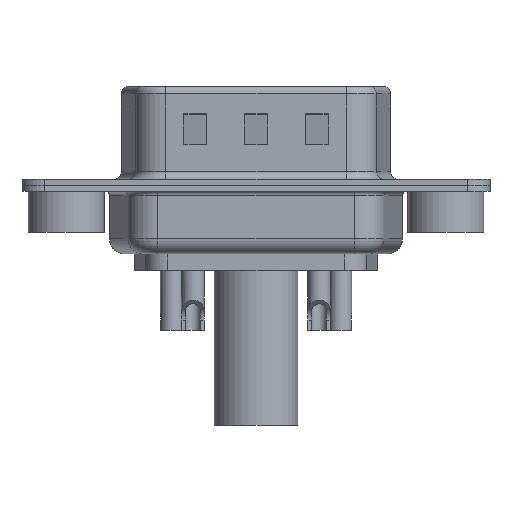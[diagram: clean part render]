
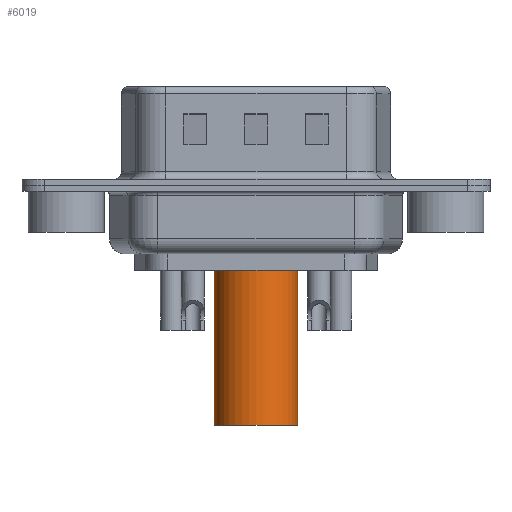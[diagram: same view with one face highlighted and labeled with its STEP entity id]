
A CAD part, front view. The second image highlights one B-rep face of the part: STEP entity #6019.
In plain terms, the highlighted cylindrical face has radius 2.75 mm (diameter 5.5 mm), a partial arc.
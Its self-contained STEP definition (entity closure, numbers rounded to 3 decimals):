
#154 = LINE ( 'NONE', #9573, #10077 ) ;
#379 = LINE ( 'NONE', #12700, #9889 ) ;
#721 = LINE ( 'NONE', #5029, #2576 ) ;
#1055 = CARTESIAN_POINT ( 'NONE',  ( 2.75, 0., -7.764 ) ) ;
#1066 = CARTESIAN_POINT ( 'NONE',  ( -2.75, 0., 1.5 ) ) ;
#1261 = VERTEX_POINT ( 'NONE', #1055 ) ;
#1787 = CYLINDRICAL_SURFACE ( 'NONE', #6380, 2.75 ) ;
#2061 = VERTEX_POINT ( 'NONE', #14835 ) ;
#2210 = DIRECTION ( 'NONE',  ( 1., 0., 0. ) ) ;
#2412 = VERTEX_POINT ( 'NONE', #3346 ) ;
#2435 = CARTESIAN_POINT ( 'NONE',  ( 0., 0., -8.7 ) ) ;
#2576 = VECTOR ( 'NONE', #14146, 1000. ) ;
#3346 = CARTESIAN_POINT ( 'NONE',  ( -2.75, 0., -7.764 ) ) ;
#3786 = CIRCLE ( 'NONE', #8337, 2.75 ) ;
#3791 = EDGE_CURVE ( 'NONE', #16579, #5732, #16949, .T. ) ;
#4065 = EDGE_CURVE ( 'NONE', #2412, #14189, #379, .T. ) ;
#4351 = EDGE_CURVE ( 'NONE', #1261, #5732, #154, .T. ) ;
#4930 = EDGE_CURVE ( 'NONE', #2412, #16579, #7479, .T. ) ;
#5029 = CARTESIAN_POINT ( 'NONE',  ( 2.75, 0., 4.234 ) ) ;
#5094 = CARTESIAN_POINT ( 'NONE',  ( 0., 0., 1.5 ) ) ;
#5098 = EDGE_LOOP ( 'NONE', ( #8766, #8073, #16456, #15986, #11383, #16383 ) ) ;
#5732 = VERTEX_POINT ( 'NONE', #8247 ) ;
#6019 = ADVANCED_FACE ( 'NONE', ( #16147 ), #1787, .T. ) ;
#6376 = DIRECTION ( 'NONE',  ( 1., 0., 0. ) ) ;
#6380 = AXIS2_PLACEMENT_3D ( 'NONE', #8889, #12108, #7188 ) ;
#6591 = EDGE_CURVE ( 'NONE', #14189, #2061, #3786, .T. ) ;
#7188 = DIRECTION ( 'NONE',  ( 1., 0., 0. ) ) ;
#7245 = CARTESIAN_POINT ( 'NONE',  ( -2.75, 0., -8.7 ) ) ;
#7479 = LINE ( 'NONE', #9342, #14003 ) ;
#7665 = AXIS2_PLACEMENT_3D ( 'NONE', #2435, #12833, #2210 ) ;
#8073 = ORIENTED_EDGE ( 'NONE', *, *, #4930, .T. ) ;
#8247 = CARTESIAN_POINT ( 'NONE',  ( 2.75, 0., -8.7 ) ) ;
#8337 = AXIS2_PLACEMENT_3D ( 'NONE', #5094, #14232, #6376 ) ;
#8502 = DIRECTION ( 'NONE',  ( 0., 0., -1. ) ) ;
#8766 = ORIENTED_EDGE ( 'NONE', *, *, #4065, .F. ) ;
#8889 = CARTESIAN_POINT ( 'NONE',  ( 0., 0., 4.234 ) ) ;
#9342 = CARTESIAN_POINT ( 'NONE',  ( -2.75, 0., -8.7 ) ) ;
#9573 = CARTESIAN_POINT ( 'NONE',  ( 2.75, 0., -8.7 ) ) ;
#9889 = VECTOR ( 'NONE', #11554, 1000. ) ;
#10077 = VECTOR ( 'NONE', #8502, 1000. ) ;
#11383 = ORIENTED_EDGE ( 'NONE', *, *, #14953, .T. ) ;
#11554 = DIRECTION ( 'NONE',  ( 0., 0., 1. ) ) ;
#12108 = DIRECTION ( 'NONE',  ( 0., 0., 1. ) ) ;
#12700 = CARTESIAN_POINT ( 'NONE',  ( -2.75, 0., 4.234 ) ) ;
#12833 = DIRECTION ( 'NONE',  ( 0., 0., 1. ) ) ;
#14003 = VECTOR ( 'NONE', #16086, 1000. ) ;
#14146 = DIRECTION ( 'NONE',  ( 0., 0., 1. ) ) ;
#14189 = VERTEX_POINT ( 'NONE', #1066 ) ;
#14232 = DIRECTION ( 'NONE',  ( 0., 0., 1. ) ) ;
#14835 = CARTESIAN_POINT ( 'NONE',  ( 2.75, 0., 1.5 ) ) ;
#14953 = EDGE_CURVE ( 'NONE', #1261, #2061, #721, .T. ) ;
#15986 = ORIENTED_EDGE ( 'NONE', *, *, #4351, .F. ) ;
#16086 = DIRECTION ( 'NONE',  ( 0., 0., -1. ) ) ;
#16147 = FACE_OUTER_BOUND ( 'NONE', #5098, .T. ) ;
#16383 = ORIENTED_EDGE ( 'NONE', *, *, #6591, .F. ) ;
#16456 = ORIENTED_EDGE ( 'NONE', *, *, #3791, .T. ) ;
#16579 = VERTEX_POINT ( 'NONE', #7245 ) ;
#16949 = CIRCLE ( 'NONE', #7665, 2.75 ) ;
